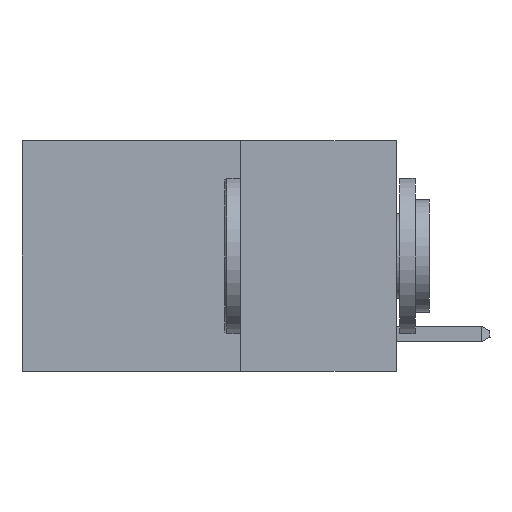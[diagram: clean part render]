
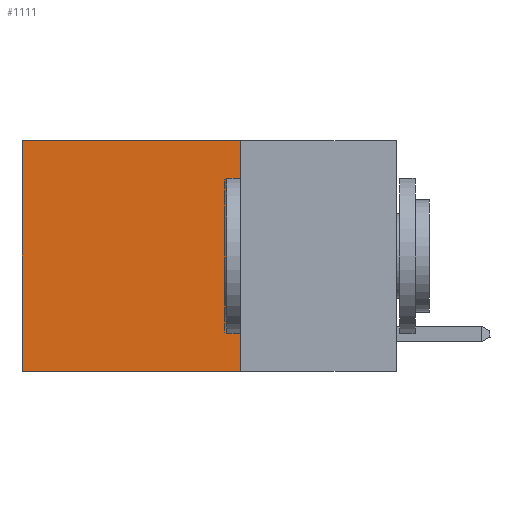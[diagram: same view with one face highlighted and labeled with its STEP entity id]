
A CAD part, left-side view. The second image highlights one B-rep face of the part: STEP entity #1111.
In plain terms, the highlighted planar face has unit normal (-1, 0, 0).
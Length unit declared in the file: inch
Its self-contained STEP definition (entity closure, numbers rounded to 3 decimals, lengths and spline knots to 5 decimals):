
#402 = ORIENTED_EDGE ( 'NONE', *, *, #5290, .T. ) ;
#438 = ORIENTED_EDGE ( 'NONE', *, *, #1672, .F. ) ;
#489 = ORIENTED_EDGE ( 'NONE', *, *, #9379, .F. ) ;
#514 = ORIENTED_EDGE ( 'NONE', *, *, #7084, .T. ) ;
#556 = CARTESIAN_POINT ( 'NONE',  ( 0.2625, 0.25, -0.37 ) ) ;
#699 = DIRECTION ( 'NONE',  ( 0., 0., -1. ) ) ;
#1068 = FACE_OUTER_BOUND ( 'NONE', #2561, .T. ) ;
#1102 = LINE ( 'NONE', #10883, #9289 ) ;
#1111 = ADVANCED_FACE ( 'NONE', ( #1068 ), #3508, .F. ) ;
#1672 = EDGE_CURVE ( 'NONE', #5392, #9512, #4787, .T. ) ;
#2482 = VECTOR ( 'NONE', #699, 39.37008 ) ;
#2561 = EDGE_LOOP ( 'NONE', ( #402, #438, #489, #514 ) ) ;
#2776 = VECTOR ( 'NONE', #11066, 39.37008 ) ;
#3214 = DIRECTION ( 'NONE',  ( 0., 0., -1. ) ) ;
#3240 = DIRECTION ( 'NONE',  ( 1., 0., 0. ) ) ;
#3393 = CARTESIAN_POINT ( 'NONE',  ( 0.2625, 0.25, 0. ) ) ;
#3508 = PLANE ( 'NONE',  #7587 ) ;
#4617 = DIRECTION ( 'NONE',  ( 0., 0., -1. ) ) ;
#4787 = LINE ( 'NONE', #556, #13050 ) ;
#4900 = VERTEX_POINT ( 'NONE', #13421 ) ;
#5290 = EDGE_CURVE ( 'NONE', #10188, #9512, #7810, .T. ) ;
#5392 = VERTEX_POINT ( 'NONE', #13414 ) ;
#7084 = EDGE_CURVE ( 'NONE', #4900, #10188, #13504, .T. ) ;
#7150 = CARTESIAN_POINT ( 'NONE',  ( 0.2625, 0.6, 0. ) ) ;
#7587 = AXIS2_PLACEMENT_3D ( 'NONE', #3393, #3240, #3214 ) ;
#7810 = LINE ( 'NONE', #7150, #2482 ) ;
#7939 = CARTESIAN_POINT ( 'NONE',  ( 0.2625, 0.25, 0. ) ) ;
#9289 = VECTOR ( 'NONE', #4617, 39.37008 ) ;
#9379 = EDGE_CURVE ( 'NONE', #4900, #5392, #1102, .T. ) ;
#9512 = VERTEX_POINT ( 'NONE', #11064 ) ;
#10188 = VERTEX_POINT ( 'NONE', #12188 ) ;
#10548 = DIRECTION ( 'NONE',  ( 0., 1., 0. ) ) ;
#10883 = CARTESIAN_POINT ( 'NONE',  ( 0.2625, 0.25, 0. ) ) ;
#11064 = CARTESIAN_POINT ( 'NONE',  ( 0.2625, 0.6, -0.37 ) ) ;
#11066 = DIRECTION ( 'NONE',  ( 0., 1., 0. ) ) ;
#12188 = CARTESIAN_POINT ( 'NONE',  ( 0.2625, 0.6, 0. ) ) ;
#13050 = VECTOR ( 'NONE', #10548, 39.37008 ) ;
#13414 = CARTESIAN_POINT ( 'NONE',  ( 0.2625, 0.25, -0.37 ) ) ;
#13421 = CARTESIAN_POINT ( 'NONE',  ( 0.2625, 0.25, 0. ) ) ;
#13504 = LINE ( 'NONE', #7939, #2776 ) ;
